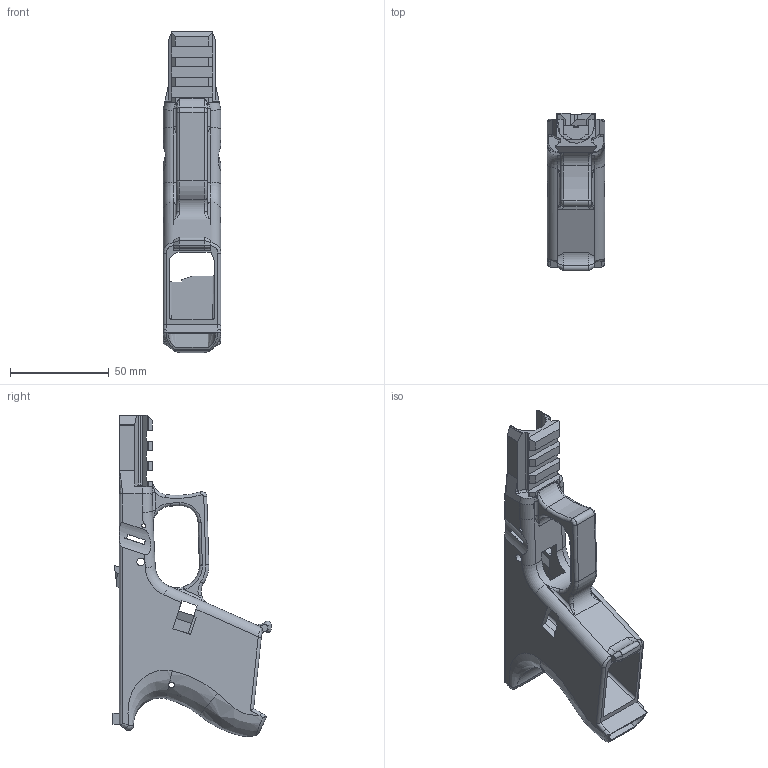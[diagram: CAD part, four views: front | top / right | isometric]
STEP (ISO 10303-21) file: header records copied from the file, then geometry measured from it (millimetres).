
FILE_DESCRIPTION(/* description */ (''),/* implementation_level */ '2;1');
FILE_NAME(/* name */ 'W26-Frame.step',/* time_stamp */ '2019-06-05T21:29:54-05:00',/* author */ (''),/* organization */ (''),/* preprocessor_version */ 'ST-DEVELOPER v18',/* originating_system */ 'Autodesk Translation Framework v8.2.0.1029',/* authorisation */ '');
FILE_SCHEMA (('AUTOMOTIVE_DESIGN { 1 0 10303 214 3 1 1 }'));
Length unit declared in the file: millimetre
Products named in the file (1): G26 Frame split
Bounding box: 29.21 x 80.11 x 162.87 mm (x, y, z)
Volume: 70000.7 mm3; surface area: 40038.3 mm2
Topology: 1 solids, 2 shells, 415 faces, 1196 edges, 761 vertices
Faces by surface type: plane 243, cylinder 97, bspline 59, torus 16
Full cylindrical faces by diameter (mm): 1.524 x1, 2 x3, 2.997 x2, 3.6 x1, 3.962 x2
Entity records: 17843 total; most frequent: CARTESIAN_POINT 7141, ORIENTED_EDGE 2376, DIRECTION 2079, EDGE_CURVE 1188, LINE 771, VECTOR 771, VERTEX_POINT 761, AXIS2_PLACEMENT_3D 654
